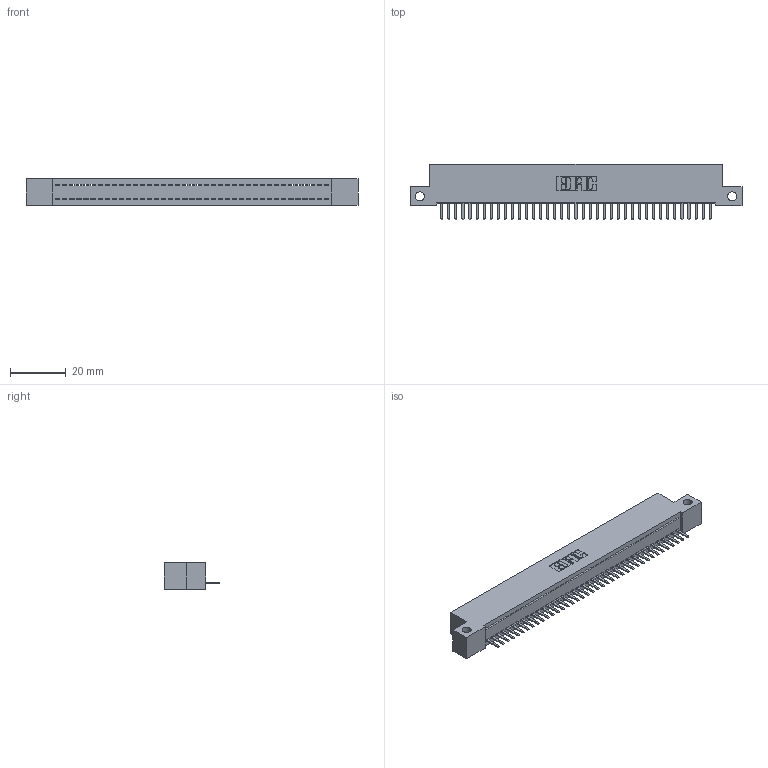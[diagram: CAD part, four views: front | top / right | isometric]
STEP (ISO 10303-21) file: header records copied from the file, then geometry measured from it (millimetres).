
FILE_DESCRIPTION (( 'STEP AP203' ), '1' );
FILE_NAME ('342-039-520-112.STEP', '2018-08-11T23:09:08', ( '' ), ( '' ), 'SwSTEP 2.0', 'SolidWorks 2016', '' );
FILE_SCHEMA (( 'CONFIG_CONTROL_DESIGN' ));
Length unit declared in the file: inch
Products named in the file (3): 345-292-001_345-293-120; 342-039-520-112; 342 Part_Side Mount
Assembly tree (40 placements, depth 2):
  342-039-520-112
    342 Part_Side Mount
    345-292-001_345-293-120  x39
Bounding box: 119.38 x 20.02 x 9.4 mm (x, y, z)
Volume: 10270.1 mm3; surface area: 14503.2 mm2
Topology: 40 solids, 40 shells, 2528 faces, 7475 edges, 4878 vertices
Faces by surface type: plane 1782, cylinder 746
Entity records: 24215 total; most frequent: CARTESIAN_POINT 4195, ORIENTED_EDGE 4158, DIRECTION 3533, EDGE_CURVE 2079, LINE 1947, VECTOR 1947, VERTEX_POINT 1382, AXIS2_PLACEMENT_3D 793
